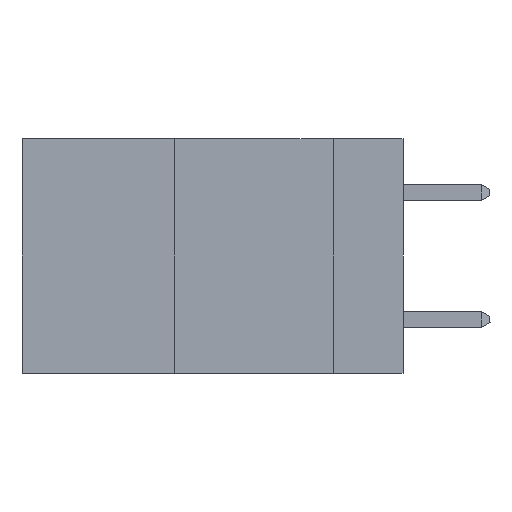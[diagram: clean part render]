
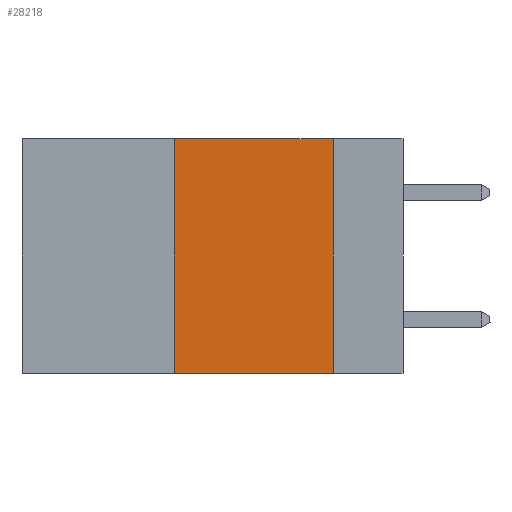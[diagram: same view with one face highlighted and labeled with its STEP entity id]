
A CAD part, left-side view. The second image highlights one B-rep face of the part: STEP entity #28218.
In plain terms, the highlighted planar face has unit normal (-1, 0, 0).
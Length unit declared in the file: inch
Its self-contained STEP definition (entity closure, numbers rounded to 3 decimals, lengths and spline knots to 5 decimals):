
#540 = FACE_OUTER_BOUND ( 'NONE', #9316, .T. ) ;
#588 = VERTEX_POINT ( 'NONE', #21364 ) ;
#863 = EDGE_CURVE ( 'NONE', #588, #13128, #939, .T. ) ;
#939 = LINE ( 'NONE', #22192, #17103 ) ;
#1017 = DIRECTION ( 'NONE',  ( 0., -1., 0. ) ) ;
#5410 = DIRECTION ( 'NONE',  ( 0., 0., -1. ) ) ;
#5698 = DIRECTION ( 'NONE',  ( 0., 0., -1. ) ) ;
#6958 = LINE ( 'NONE', #10841, #27783 ) ;
#7152 = CARTESIAN_POINT ( 'NONE',  ( 0., 0.6, 0. ) ) ;
#8239 = VECTOR ( 'NONE', #5698, 39.37008 ) ;
#8429 = CARTESIAN_POINT ( 'NONE',  ( 0., 0.11, 0. ) ) ;
#9316 = EDGE_LOOP ( 'NONE', ( #12316, #17442, #15905, #22700 ) ) ;
#10841 = CARTESIAN_POINT ( 'NONE',  ( 0., 0.6, -0.37 ) ) ;
#11279 = DIRECTION ( 'NONE',  ( 0., -1., 0. ) ) ;
#12316 = ORIENTED_EDGE ( 'NONE', *, *, #23267, .F. ) ;
#12474 = EDGE_CURVE ( 'NONE', #588, #15228, #6958, .T. ) ;
#13128 = VERTEX_POINT ( 'NONE', #20705 ) ;
#14051 = PLANE ( 'NONE',  #18787 ) ;
#15228 = VERTEX_POINT ( 'NONE', #26230 ) ;
#15750 = DIRECTION ( 'NONE',  ( 0., 0., 1. ) ) ;
#15905 = ORIENTED_EDGE ( 'NONE', *, *, #863, .F. ) ;
#16401 = VECTOR ( 'NONE', #1017, 39.37008 ) ;
#17103 = VECTOR ( 'NONE', #15750, 39.37008 ) ;
#17442 = ORIENTED_EDGE ( 'NONE', *, *, #20465, .F. ) ;
#18342 = DIRECTION ( 'NONE',  ( 1., 0., 0. ) ) ;
#18390 = LINE ( 'NONE', #20688, #16401 ) ;
#18787 = AXIS2_PLACEMENT_3D ( 'NONE', #7152, #18342, #5410 ) ;
#20465 = EDGE_CURVE ( 'NONE', #13128, #24100, #18390, .T. ) ;
#20688 = CARTESIAN_POINT ( 'NONE',  ( 0., 0.6, 0. ) ) ;
#20705 = CARTESIAN_POINT ( 'NONE',  ( 0., 0.36, 0. ) ) ;
#21364 = CARTESIAN_POINT ( 'NONE',  ( 0., 0.36, -0.37 ) ) ;
#22192 = CARTESIAN_POINT ( 'NONE',  ( 0., 0.36, 0. ) ) ;
#22700 = ORIENTED_EDGE ( 'NONE', *, *, #12474, .T. ) ;
#23267 = EDGE_CURVE ( 'NONE', #24100, #15228, #23513, .T. ) ;
#23513 = LINE ( 'NONE', #8429, #8239 ) ;
#24100 = VERTEX_POINT ( 'NONE', #25821 ) ;
#25821 = CARTESIAN_POINT ( 'NONE',  ( 0., 0.11, 0. ) ) ;
#26230 = CARTESIAN_POINT ( 'NONE',  ( 0., 0.11, -0.37 ) ) ;
#27783 = VECTOR ( 'NONE', #11279, 39.37008 ) ;
#28218 = ADVANCED_FACE ( 'NONE', ( #540 ), #14051, .F. ) ;
